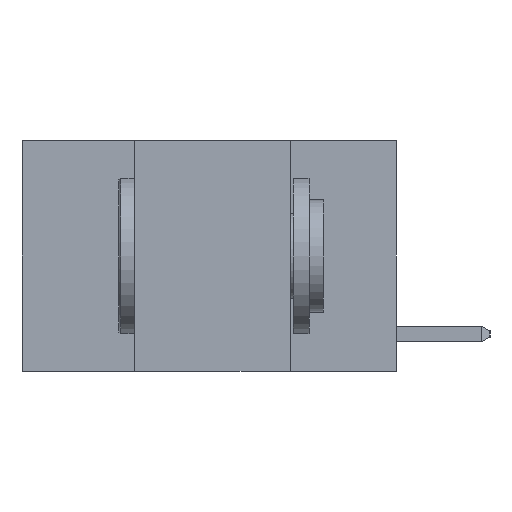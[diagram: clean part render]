
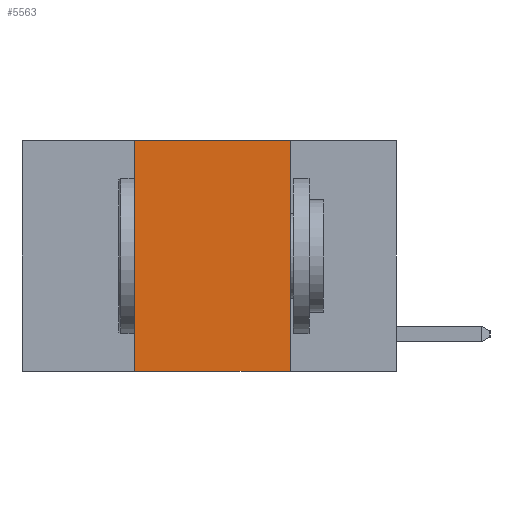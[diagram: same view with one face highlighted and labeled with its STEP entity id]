
A CAD part, left-side view. The second image highlights one B-rep face of the part: STEP entity #5563.
In plain terms, the highlighted planar face has unit normal (-1, 0, 0).
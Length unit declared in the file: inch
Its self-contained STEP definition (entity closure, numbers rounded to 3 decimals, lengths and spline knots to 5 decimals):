
#170 = CARTESIAN_POINT ( 'NONE',  ( 0., 0.17, 0. ) ) ;
#252 = CARTESIAN_POINT ( 'NONE',  ( 0., 0.42, 0. ) ) ;
#2277 = ORIENTED_EDGE ( 'NONE', *, *, #10141, .T. ) ;
#2470 = ORIENTED_EDGE ( 'NONE', *, *, #9721, .F. ) ;
#2500 = VERTEX_POINT ( 'NONE', #252 ) ;
#2797 = LINE ( 'NONE', #6798, #9471 ) ;
#3052 = LINE ( 'NONE', #13280, #15993 ) ;
#3059 = EDGE_CURVE ( 'NONE', #7315, #13466, #2797, .T. ) ;
#3242 = DIRECTION ( 'NONE',  ( 0., -1., 0. ) ) ;
#3725 = FACE_OUTER_BOUND ( 'NONE', #15826, .T. ) ;
#5346 = VECTOR ( 'NONE', #11420, 39.37008 ) ;
#5517 = DIRECTION ( 'NONE',  ( 1., 0., 0. ) ) ;
#5563 = ADVANCED_FACE ( 'NONE', ( #3725 ), #10515, .F. ) ;
#5813 = CARTESIAN_POINT ( 'NONE',  ( 0., 0.17, -0.37 ) ) ;
#6798 = CARTESIAN_POINT ( 'NONE',  ( 0., 0.17, 0. ) ) ;
#6917 = AXIS2_PLACEMENT_3D ( 'NONE', #13023, #5517, #14287 ) ;
#7311 = ORIENTED_EDGE ( 'NONE', *, *, #3059, .F. ) ;
#7315 = VERTEX_POINT ( 'NONE', #170 ) ;
#8047 = DIRECTION ( 'NONE',  ( 0., 0., -1. ) ) ;
#9471 = VECTOR ( 'NONE', #8047, 39.37008 ) ;
#9721 = EDGE_CURVE ( 'NONE', #15180, #2500, #12051, .T. ) ;
#10141 = EDGE_CURVE ( 'NONE', #15180, #13466, #12039, .T. ) ;
#10515 = PLANE ( 'NONE',  #6917 ) ;
#10870 = CARTESIAN_POINT ( 'NONE',  ( 0., 0.42, -0.37 ) ) ;
#11420 = DIRECTION ( 'NONE',  ( 0., -1., 0. ) ) ;
#11883 = CARTESIAN_POINT ( 'NONE',  ( 0., 0.42, 0. ) ) ;
#12039 = LINE ( 'NONE', #13885, #5346 ) ;
#12051 = LINE ( 'NONE', #11883, #14971 ) ;
#12906 = ORIENTED_EDGE ( 'NONE', *, *, #14580, .F. ) ;
#13023 = CARTESIAN_POINT ( 'NONE',  ( 0., 0.6, 0. ) ) ;
#13280 = CARTESIAN_POINT ( 'NONE',  ( 0., 0.6, 0. ) ) ;
#13466 = VERTEX_POINT ( 'NONE', #5813 ) ;
#13885 = CARTESIAN_POINT ( 'NONE',  ( 0., 0.6, -0.37 ) ) ;
#14287 = DIRECTION ( 'NONE',  ( 0., 0., -1. ) ) ;
#14340 = DIRECTION ( 'NONE',  ( 0., 0., 1. ) ) ;
#14580 = EDGE_CURVE ( 'NONE', #2500, #7315, #3052, .T. ) ;
#14971 = VECTOR ( 'NONE', #14340, 39.37008 ) ;
#15180 = VERTEX_POINT ( 'NONE', #10870 ) ;
#15826 = EDGE_LOOP ( 'NONE', ( #7311, #12906, #2470, #2277 ) ) ;
#15993 = VECTOR ( 'NONE', #3242, 39.37008 ) ;
